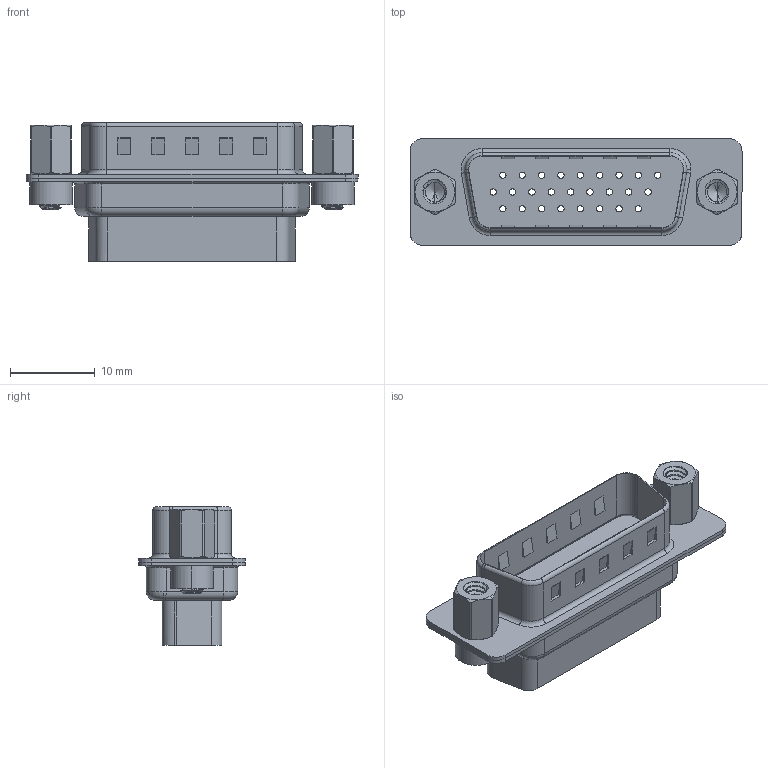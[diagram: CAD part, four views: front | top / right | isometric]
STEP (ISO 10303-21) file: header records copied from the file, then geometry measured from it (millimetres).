
FILE_DESCRIPTION (( 'STEP AP203' ), '1' );
FILE_NAME ('637-026-010-243.STEP', '2020-07-17T21:17:57', ( '' ), ( '' ), 'SwSTEP 2.0', 'SolidWorks 2020', '' );
FILE_SCHEMA (( 'CONFIG_CONTROL_DESIGN' ));
Length unit declared in the file: millimetre
Products named in the file (6): 637 4-40 Threaded Rivet; 637 Shell Rear_26 Contacts; 637 Shell Front_26 Contacts; 637 4-40 Hex Standoff; 637 Housing_26 Contacts HP; 637-026-010-243
Assembly tree (7 placements, depth 2):
  637-026-010-243
    637 Housing_26 Contacts HP
    637 Shell Front_26 Contacts
    637 Shell Rear_26 Contacts
    637 4-40 Threaded Rivet  x2
    637 4-40 Hex Standoff  x2
Bounding box: 39.2 x 12.6 x 16.4 mm (x, y, z)
Volume: 2263.4 mm3; surface area: 5604.4 mm2
Topology: 7 solids, 7 shells, 674 faces, 1673 edges, 1076 vertices
Faces by surface type: cylinder 361, plane 213, torus 50, cone 32, bspline 18
Entity records: 22043 total; most frequent: CARTESIAN_POINT 7340, DIRECTION 3059, ORIENTED_EDGE 2832, EDGE_CURVE 1416, AXIS2_PLACEMENT_3D 1202, VERTEX_POINT 911, EDGE_LOOP 727, VECTOR 655
